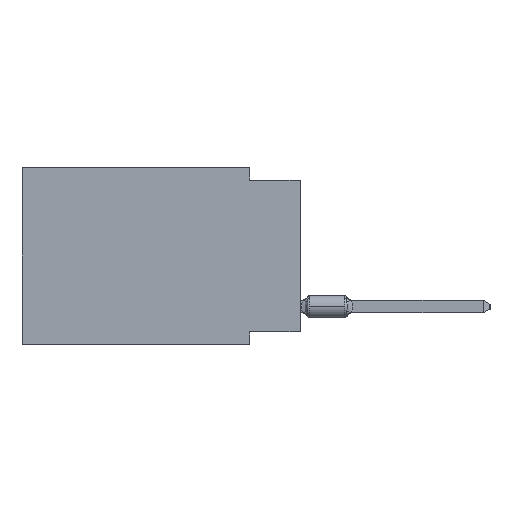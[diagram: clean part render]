
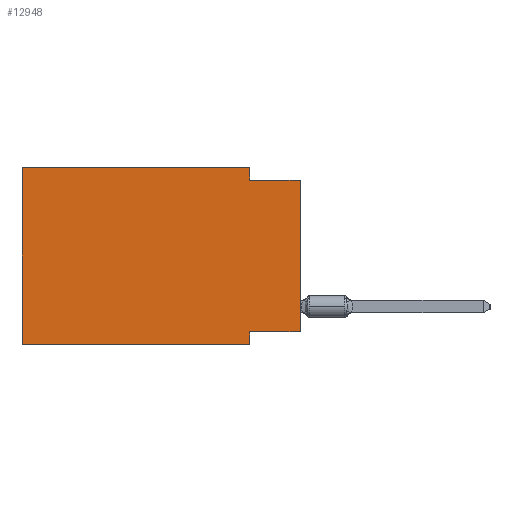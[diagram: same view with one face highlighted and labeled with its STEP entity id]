
A CAD part, left-side view. The second image highlights one B-rep face of the part: STEP entity #12948.
In plain terms, the highlighted planar face has unit normal (-1, 0, 0).
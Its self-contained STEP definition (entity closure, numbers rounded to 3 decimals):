
#1216 = LINE ( 'NONE', #74678, #7423 ) ;
#1224 = LINE ( 'NONE', #27713, #55046 ) ;
#2006 = ORIENTED_EDGE ( 'NONE', *, *, #34005, .F. ) ;
#3140 = ORIENTED_EDGE ( 'NONE', *, *, #62083, .T. ) ;
#3477 = ORIENTED_EDGE ( 'NONE', *, *, #42559, .F. ) ;
#4371 = LINE ( 'NONE', #83932, #61548 ) ;
#4621 = LINE ( 'NONE', #77645, #48100 ) ;
#4957 = LINE ( 'NONE', #77149, #84688 ) ;
#7423 = VECTOR ( 'NONE', #55094, 1000. ) ;
#8635 = CARTESIAN_POINT ( 'NONE',  ( 0., 13.97, 0. ) ) ;
#12948 = ADVANCED_FACE ( 'NONE', ( #27329 ), #29031, .F. ) ;
#14726 = DIRECTION ( 'NONE',  ( 0., -1., 0. ) ) ;
#19041 = ORIENTED_EDGE ( 'NONE', *, *, #54371, .F. ) ;
#20021 = DIRECTION ( 'NONE',  ( 0., 0., 1. ) ) ;
#20316 = CARTESIAN_POINT ( 'NONE',  ( 0., 2.54, -8.89 ) ) ;
#20699 = VERTEX_POINT ( 'NONE', #71310 ) ;
#23464 = AXIS2_PLACEMENT_3D ( 'NONE', #8635, #60825, #42115 ) ;
#23903 = DIRECTION ( 'NONE',  ( 0., 0., -1. ) ) ;
#26820 = CARTESIAN_POINT ( 'NONE',  ( 0., 0., -0.635 ) ) ;
#27329 = FACE_OUTER_BOUND ( 'NONE', #49458, .T. ) ;
#27713 = CARTESIAN_POINT ( 'NONE',  ( 0., 13.97, 0. ) ) ;
#29031 = PLANE ( 'NONE',  #23464 ) ;
#29175 = EDGE_CURVE ( 'NONE', #82636, #75502, #34728, .T. ) ;
#30098 = EDGE_CURVE ( 'NONE', #76226, #35530, #4371, .T. ) ;
#30428 = LINE ( 'NONE', #76549, #73723 ) ;
#33856 = EDGE_CURVE ( 'NONE', #82636, #68428, #1224, .T. ) ;
#34005 = EDGE_CURVE ( 'NONE', #44035, #75502, #4621, .T. ) ;
#34728 = LINE ( 'NONE', #74306, #37807 ) ;
#35530 = VERTEX_POINT ( 'NONE', #26820 ) ;
#37807 = VECTOR ( 'NONE', #14726, 1000. ) ;
#41958 = ORIENTED_EDGE ( 'NONE', *, *, #29175, .T. ) ;
#42115 = DIRECTION ( 'NONE',  ( 0., 0., -1. ) ) ;
#42559 = EDGE_CURVE ( 'NONE', #67676, #44035, #1216, .T. ) ;
#44035 = VERTEX_POINT ( 'NONE', #65903 ) ;
#48100 = VECTOR ( 'NONE', #78088, 1000. ) ;
#49458 = EDGE_LOOP ( 'NONE', ( #3140, #66058, #72901, #19041, #67979, #41958, #2006, #3477 ) ) ;
#52526 = DIRECTION ( 'NONE',  ( 0., 0., 1. ) ) ;
#53514 = CARTESIAN_POINT ( 'NONE',  ( 0., 0., 0. ) ) ;
#53556 = EDGE_CURVE ( 'NONE', #20699, #76226, #30428, .T. ) ;
#54371 = EDGE_CURVE ( 'NONE', #68428, #20699, #4957, .T. ) ;
#55046 = VECTOR ( 'NONE', #52526, 1000. ) ;
#55094 = DIRECTION ( 'NONE',  ( 0., 1., 0. ) ) ;
#59070 = CARTESIAN_POINT ( 'NONE',  ( 0., 2.54, -0.635 ) ) ;
#60825 = DIRECTION ( 'NONE',  ( 1., 0., 0. ) ) ;
#61548 = VECTOR ( 'NONE', #81061, 1000. ) ;
#62000 = VECTOR ( 'NONE', #20021, 1000. ) ;
#62083 = EDGE_CURVE ( 'NONE', #67676, #35530, #80470, .T. ) ;
#65903 = CARTESIAN_POINT ( 'NONE',  ( 0., 2.54, -8.255 ) ) ;
#66058 = ORIENTED_EDGE ( 'NONE', *, *, #30098, .F. ) ;
#67676 = VERTEX_POINT ( 'NONE', #68759 ) ;
#67979 = ORIENTED_EDGE ( 'NONE', *, *, #33856, .F. ) ;
#68428 = VERTEX_POINT ( 'NONE', #75093 ) ;
#68606 = DIRECTION ( 'NONE',  ( 0., -1., 0. ) ) ;
#68759 = CARTESIAN_POINT ( 'NONE',  ( 0., 0., -8.255 ) ) ;
#71310 = CARTESIAN_POINT ( 'NONE',  ( 0., 2.54, 0. ) ) ;
#72901 = ORIENTED_EDGE ( 'NONE', *, *, #53556, .F. ) ;
#73723 = VECTOR ( 'NONE', #23903, 1000. ) ;
#74306 = CARTESIAN_POINT ( 'NONE',  ( 0., 13.97, -8.89 ) ) ;
#74678 = CARTESIAN_POINT ( 'NONE',  ( 0., 0., -8.255 ) ) ;
#75093 = CARTESIAN_POINT ( 'NONE',  ( 0., 13.97, 0. ) ) ;
#75502 = VERTEX_POINT ( 'NONE', #20316 ) ;
#76226 = VERTEX_POINT ( 'NONE', #59070 ) ;
#76549 = CARTESIAN_POINT ( 'NONE',  ( 0., 2.54, 0. ) ) ;
#77149 = CARTESIAN_POINT ( 'NONE',  ( 0., 13.97, 0. ) ) ;
#77601 = CARTESIAN_POINT ( 'NONE',  ( 0., 13.97, -8.89 ) ) ;
#77645 = CARTESIAN_POINT ( 'NONE',  ( 0., 2.54, -8.89 ) ) ;
#78088 = DIRECTION ( 'NONE',  ( 0., 0., -1. ) ) ;
#80470 = LINE ( 'NONE', #53514, #62000 ) ;
#81061 = DIRECTION ( 'NONE',  ( 0., -1., 0. ) ) ;
#82636 = VERTEX_POINT ( 'NONE', #77601 ) ;
#83932 = CARTESIAN_POINT ( 'NONE',  ( 0., 0., -0.635 ) ) ;
#84688 = VECTOR ( 'NONE', #68606, 1000. ) ;
